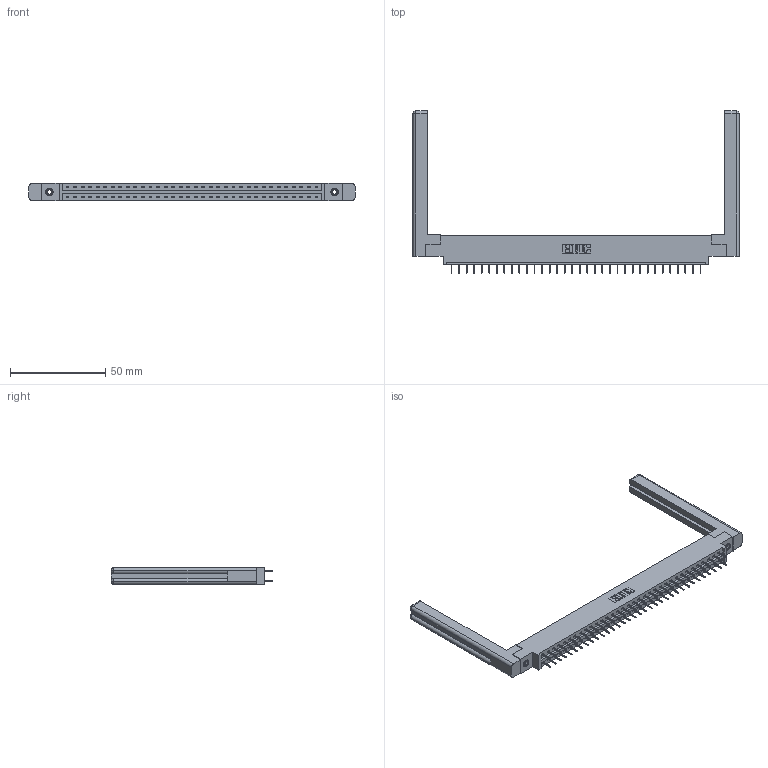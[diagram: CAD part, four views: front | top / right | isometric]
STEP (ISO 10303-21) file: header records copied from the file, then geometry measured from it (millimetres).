
FILE_DESCRIPTION (( 'STEP AP203' ), '1' );
FILE_NAME ('337-068-524-858.STEP', '2019-10-12T02:04:19', ( '' ), ( '' ), 'SwSTEP 2.0', 'SolidWorks 2016', '' );
FILE_SCHEMA (( 'CONFIG_CONTROL_DESIGN' ));
Length unit declared in the file: inch
Products named in the file (5): 337 Part_0.170 Offset - 0.156 Dia-TI; 345-250-001_345-250-001-102; 307-220-058; 345-292-001_345-293-124; 337-068-524-858
Assembly tree (73 placements, depth 2):
  337-068-524-858
    337 Part_0.170 Offset - 0.156 Dia-TI
    345-292-001_345-293-124  x68
    345-250-001_345-250-001-102  x2
    307-220-058  x2
Bounding box: 171.35 x 85.1 x 9.4 mm (x, y, z)
Volume: 24873.5 mm3; surface area: 24803.3 mm2
Topology: 73 solids, 73 shells, 4204 faces, 11897 edges, 7646 vertices
Faces by surface type: plane 3150, cylinder 1030, cone 12, torus 12
Entity records: 30236 total; most frequent: CARTESIAN_POINT 5109, ORIENTED_EDGE 4984, DIRECTION 4376, EDGE_CURVE 2492, LINE 2320, VECTOR 2320, VERTEX_POINT 1650, AXIS2_PLACEMENT_3D 1028
